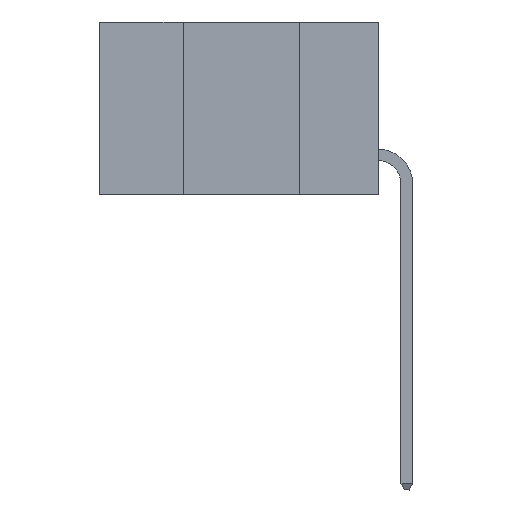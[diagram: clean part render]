
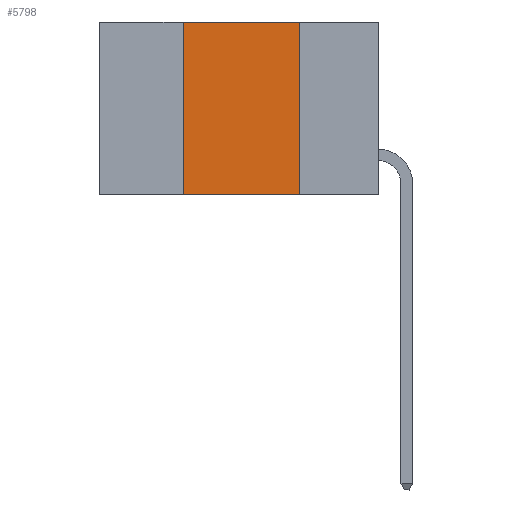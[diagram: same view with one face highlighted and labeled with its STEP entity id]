
A CAD part, left-side view. The second image highlights one B-rep face of the part: STEP entity #5798.
In plain terms, the highlighted planar face has unit normal (-1, 0, 0).
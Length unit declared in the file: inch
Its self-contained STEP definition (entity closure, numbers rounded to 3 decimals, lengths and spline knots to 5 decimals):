
#301 = LINE ( 'NONE', #2524, #13213 ) ;
#537 = CARTESIAN_POINT ( 'NONE',  ( 0., 0.17, 0. ) ) ;
#635 = CARTESIAN_POINT ( 'NONE',  ( 0., 0.17, -0.37 ) ) ;
#923 = DIRECTION ( 'NONE',  ( 1., 0., 0. ) ) ;
#983 = PLANE ( 'NONE',  #3046 ) ;
#1251 = VERTEX_POINT ( 'NONE', #7639 ) ;
#1519 = CARTESIAN_POINT ( 'NONE',  ( 0., 0.17, -0.37 ) ) ;
#1587 = VERTEX_POINT ( 'NONE', #537 ) ;
#1762 = LINE ( 'NONE', #635, #14494 ) ;
#2107 = VERTEX_POINT ( 'NONE', #1519 ) ;
#2123 = CARTESIAN_POINT ( 'NONE',  ( 0., 0.42, 0. ) ) ;
#2484 = DIRECTION ( 'NONE',  ( 0., 0., 1. ) ) ;
#2524 = CARTESIAN_POINT ( 'NONE',  ( 0., 0.6, -0.37 ) ) ;
#2951 = VECTOR ( 'NONE', #2484, 39.37008 ) ;
#3046 = AXIS2_PLACEMENT_3D ( 'NONE', #7565, #923, #4361 ) ;
#3067 = VERTEX_POINT ( 'NONE', #2123 ) ;
#3282 = ORIENTED_EDGE ( 'NONE', *, *, #4715, .F. ) ;
#3603 = DIRECTION ( 'NONE',  ( 0., -1., 0. ) ) ;
#3649 = ORIENTED_EDGE ( 'NONE', *, *, #6355, .F. ) ;
#3683 = LINE ( 'NONE', #9276, #2951 ) ;
#4361 = DIRECTION ( 'NONE',  ( 0., 0., -1. ) ) ;
#4715 = EDGE_CURVE ( 'NONE', #1587, #2107, #1762, .T. ) ;
#4880 = DIRECTION ( 'NONE',  ( 0., -1., 0. ) ) ;
#5798 = ADVANCED_FACE ( 'NONE', ( #14655 ), #983, .F. ) ;
#6352 = EDGE_CURVE ( 'NONE', #3067, #1587, #8090, .T. ) ;
#6355 = EDGE_CURVE ( 'NONE', #1251, #3067, #3683, .T. ) ;
#7226 = ORIENTED_EDGE ( 'NONE', *, *, #6352, .F. ) ;
#7565 = CARTESIAN_POINT ( 'NONE',  ( 0., 0.6, 0. ) ) ;
#7639 = CARTESIAN_POINT ( 'NONE',  ( 0., 0.42, -0.37 ) ) ;
#8090 = LINE ( 'NONE', #10389, #9379 ) ;
#8376 = EDGE_CURVE ( 'NONE', #1251, #2107, #301, .T. ) ;
#9037 = DIRECTION ( 'NONE',  ( 0., 0., -1. ) ) ;
#9276 = CARTESIAN_POINT ( 'NONE',  ( 0., 0.42, -0.37 ) ) ;
#9310 = ORIENTED_EDGE ( 'NONE', *, *, #8376, .T. ) ;
#9379 = VECTOR ( 'NONE', #3603, 39.37008 ) ;
#10389 = CARTESIAN_POINT ( 'NONE',  ( 0., 0.6, 0. ) ) ;
#13213 = VECTOR ( 'NONE', #4880, 39.37008 ) ;
#14210 = EDGE_LOOP ( 'NONE', ( #3282, #7226, #3649, #9310 ) ) ;
#14494 = VECTOR ( 'NONE', #9037, 39.37008 ) ;
#14655 = FACE_OUTER_BOUND ( 'NONE', #14210, .T. ) ;
